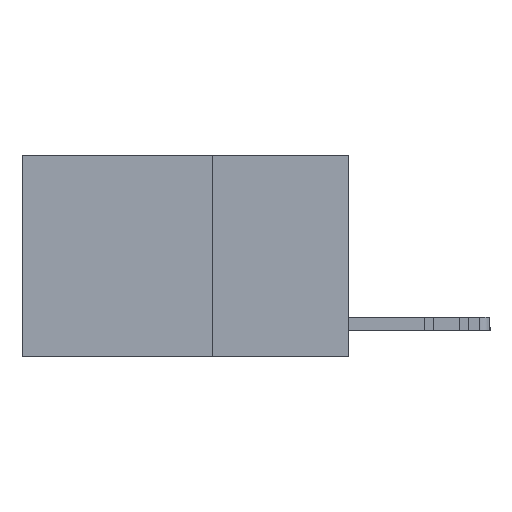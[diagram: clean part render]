
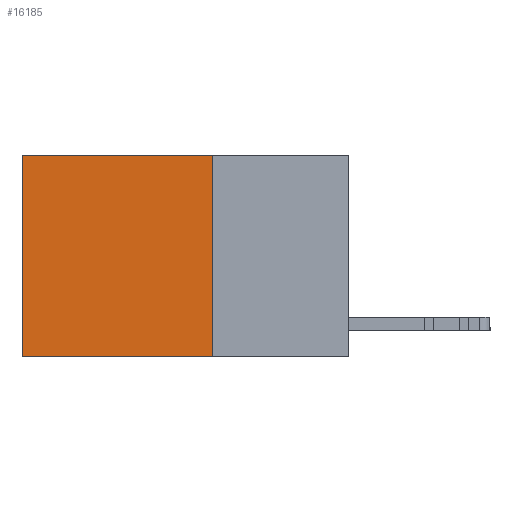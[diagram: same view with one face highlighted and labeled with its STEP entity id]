
A CAD part, left-side view. The second image highlights one B-rep face of the part: STEP entity #16185.
In plain terms, the highlighted planar face has unit normal (-1, 0, 0).
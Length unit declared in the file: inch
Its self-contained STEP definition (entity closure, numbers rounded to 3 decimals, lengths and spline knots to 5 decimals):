
#323 = DIRECTION ( 'NONE',  ( 0., 0., -1. ) ) ;
#1712 = CARTESIAN_POINT ( 'NONE',  ( 0.2625, 0.6, 0. ) ) ;
#2711 = ORIENTED_EDGE ( 'NONE', *, *, #22484, .F. ) ;
#2792 = CARTESIAN_POINT ( 'NONE',  ( 0.2625, 0.25, 0. ) ) ;
#3921 = VERTEX_POINT ( 'NONE', #1712 ) ;
#4825 = EDGE_CURVE ( 'NONE', #3921, #25250, #7321, .T. ) ;
#4936 = DIRECTION ( 'NONE',  ( 0., 0., -1. ) ) ;
#5003 = ORIENTED_EDGE ( 'NONE', *, *, #16812, .F. ) ;
#5056 = CARTESIAN_POINT ( 'NONE',  ( 0.2625, 0.25, -0.37 ) ) ;
#5247 = DIRECTION ( 'NONE',  ( 1., 0., 0. ) ) ;
#5973 = AXIS2_PLACEMENT_3D ( 'NONE', #2792, #5247, #4936 ) ;
#6574 = VERTEX_POINT ( 'NONE', #29844 ) ;
#7321 = LINE ( 'NONE', #29981, #25400 ) ;
#8078 = EDGE_LOOP ( 'NONE', ( #11399, #2711, #5003, #8722 ) ) ;
#8467 = VECTOR ( 'NONE', #323, 39.37008 ) ;
#8722 = ORIENTED_EDGE ( 'NONE', *, *, #9998, .T. ) ;
#9998 = EDGE_CURVE ( 'NONE', #6574, #3921, #27741, .T. ) ;
#11399 = ORIENTED_EDGE ( 'NONE', *, *, #4825, .T. ) ;
#13078 = DIRECTION ( 'NONE',  ( 0., 1., 0. ) ) ;
#16185 = ADVANCED_FACE ( 'NONE', ( #26722 ), #29076, .F. ) ;
#16250 = VECTOR ( 'NONE', #17713, 39.37008 ) ;
#16810 = LINE ( 'NONE', #5056, #22846 ) ;
#16812 = EDGE_CURVE ( 'NONE', #6574, #29641, #25706, .T. ) ;
#17713 = DIRECTION ( 'NONE',  ( 0., 1., 0. ) ) ;
#19073 = DIRECTION ( 'NONE',  ( 0., 0., -1. ) ) ;
#22484 = EDGE_CURVE ( 'NONE', #29641, #25250, #16810, .T. ) ;
#22523 = CARTESIAN_POINT ( 'NONE',  ( 0.2625, 0.25, -0.37 ) ) ;
#22846 = VECTOR ( 'NONE', #13078, 39.37008 ) ;
#23248 = CARTESIAN_POINT ( 'NONE',  ( 0.2625, 0.25, 0. ) ) ;
#25250 = VERTEX_POINT ( 'NONE', #28668 ) ;
#25400 = VECTOR ( 'NONE', #19073, 39.37008 ) ;
#25706 = LINE ( 'NONE', #23248, #8467 ) ;
#26722 = FACE_OUTER_BOUND ( 'NONE', #8078, .T. ) ;
#27741 = LINE ( 'NONE', #30091, #16250 ) ;
#28668 = CARTESIAN_POINT ( 'NONE',  ( 0.2625, 0.6, -0.37 ) ) ;
#29076 = PLANE ( 'NONE',  #5973 ) ;
#29641 = VERTEX_POINT ( 'NONE', #22523 ) ;
#29844 = CARTESIAN_POINT ( 'NONE',  ( 0.2625, 0.25, 0. ) ) ;
#29981 = CARTESIAN_POINT ( 'NONE',  ( 0.2625, 0.6, 0. ) ) ;
#30091 = CARTESIAN_POINT ( 'NONE',  ( 0.2625, 0.25, 0. ) ) ;
